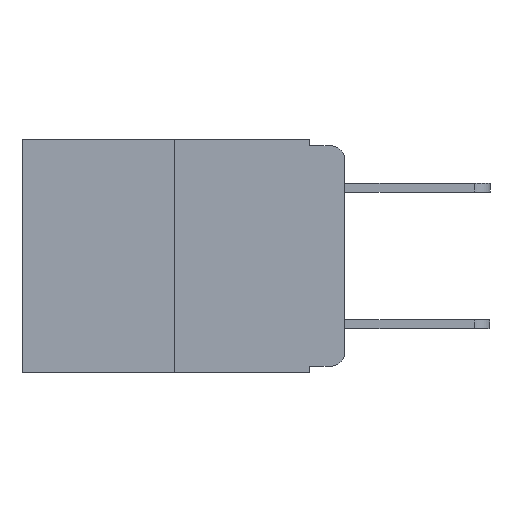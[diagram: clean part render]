
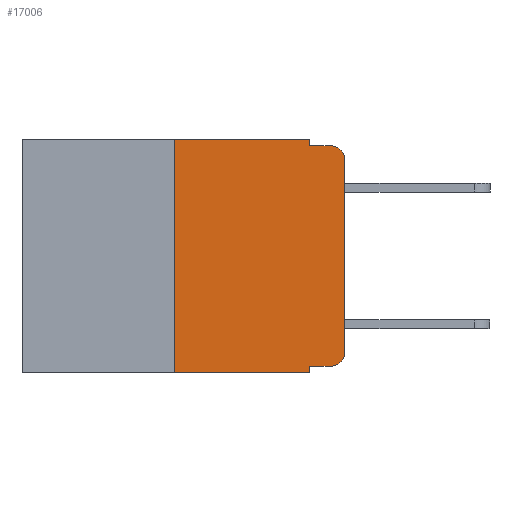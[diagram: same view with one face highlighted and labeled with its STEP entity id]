
A CAD part, left-side view. The second image highlights one B-rep face of the part: STEP entity #17006.
In plain terms, the highlighted planar face has unit normal (-1, 0, 0).
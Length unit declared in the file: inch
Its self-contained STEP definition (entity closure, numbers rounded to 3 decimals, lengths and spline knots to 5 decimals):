
#28 = DIRECTION ( 'NONE',  ( 0., 0., 1. ) ) ;
#398 = EDGE_CURVE ( 'NONE', #14996, #5496, #13515, .T. ) ;
#632 = CARTESIAN_POINT ( 'NONE',  ( 0., 0., 0. ) ) ;
#847 = EDGE_CURVE ( 'NONE', #13407, #10683, #22896, .T. ) ;
#879 = CARTESIAN_POINT ( 'NONE',  ( 0., 0.051, 0. ) ) ;
#947 = ORIENTED_EDGE ( 'NONE', *, *, #847, .F. ) ;
#1646 = VECTOR ( 'NONE', #8647, 39.37008 ) ;
#2410 = CARTESIAN_POINT ( 'NONE',  ( 0., 0.02, -0.313 ) ) ;
#2514 = AXIS2_PLACEMENT_3D ( 'NONE', #2410, #15236, #4352 ) ;
#2531 = CARTESIAN_POINT ( 'NONE',  ( 0., 0.473, -0.343 ) ) ;
#2875 = CARTESIAN_POINT ( 'NONE',  ( 0., 0.25, 0. ) ) ;
#2968 = VERTEX_POINT ( 'NONE', #19376 ) ;
#3400 = PLANE ( 'NONE',  #21052 ) ;
#3443 = EDGE_CURVE ( 'NONE', #10683, #14114, #18419, .T. ) ;
#3958 = VECTOR ( 'NONE', #11970, 39.37008 ) ;
#4352 = DIRECTION ( 'NONE',  ( 0., 0., -1. ) ) ;
#4741 = EDGE_CURVE ( 'NONE', #15230, #14114, #15304, .T. ) ;
#5105 = VECTOR ( 'NONE', #18963, 39.37008 ) ;
#5323 = DIRECTION ( 'NONE',  ( 0., 0., -1. ) ) ;
#5496 = VERTEX_POINT ( 'NONE', #22083 ) ;
#5988 = EDGE_CURVE ( 'NONE', #2968, #15230, #6943, .T. ) ;
#6168 = CARTESIAN_POINT ( 'NONE',  ( 0., 0.051, -0.333 ) ) ;
#6943 = LINE ( 'NONE', #632, #15933 ) ;
#8115 = CARTESIAN_POINT ( 'NONE',  ( 0., 0.051, -0.01 ) ) ;
#8647 = DIRECTION ( 'NONE',  ( 0., 0., 1. ) ) ;
#9089 = EDGE_CURVE ( 'NONE', #20933, #13407, #13251, .T. ) ;
#10307 = ORIENTED_EDGE ( 'NONE', *, *, #4741, .T. ) ;
#10341 = VECTOR ( 'NONE', #21793, 39.37008 ) ;
#10683 = VERTEX_POINT ( 'NONE', #8115 ) ;
#10888 = LINE ( 'NONE', #14692, #10341 ) ;
#11970 = DIRECTION ( 'NONE',  ( 0., -1., 0. ) ) ;
#12335 = CARTESIAN_POINT ( 'NONE',  ( 0., 0.473, 0. ) ) ;
#12563 = ORIENTED_EDGE ( 'NONE', *, *, #23173, .F. ) ;
#12940 = VECTOR ( 'NONE', #14552, 39.37008 ) ;
#13251 = LINE ( 'NONE', #12335, #22099 ) ;
#13407 = VERTEX_POINT ( 'NONE', #23140 ) ;
#13515 = LINE ( 'NONE', #2531, #12940 ) ;
#13629 = CIRCLE ( 'NONE', #2514, 0.02 ) ;
#14063 = VECTOR ( 'NONE', #23509, 39.37008 ) ;
#14114 = VERTEX_POINT ( 'NONE', #19898 ) ;
#14155 = DIRECTION ( 'NONE',  ( 0., -1., 0. ) ) ;
#14428 = CARTESIAN_POINT ( 'NONE',  ( 0., 0., -0.03 ) ) ;
#14552 = DIRECTION ( 'NONE',  ( 0., -1., 0. ) ) ;
#14692 = CARTESIAN_POINT ( 'NONE',  ( 0., 0.051, -0.333 ) ) ;
#14815 = ORIENTED_EDGE ( 'NONE', *, *, #16123, .T. ) ;
#14996 = VERTEX_POINT ( 'NONE', #22612 ) ;
#15088 = ORIENTED_EDGE ( 'NONE', *, *, #3443, .F. ) ;
#15230 = VERTEX_POINT ( 'NONE', #14428 ) ;
#15236 = DIRECTION ( 'NONE',  ( -1., 0., 0. ) ) ;
#15304 = CIRCLE ( 'NONE', #21744, 0.02 ) ;
#15377 = CARTESIAN_POINT ( 'NONE',  ( 0., 0.051, 0. ) ) ;
#15645 = CARTESIAN_POINT ( 'NONE',  ( 0., 0.02, -0.333 ) ) ;
#15814 = CARTESIAN_POINT ( 'NONE',  ( 0., 0.25, 0. ) ) ;
#15933 = VECTOR ( 'NONE', #28, 39.37008 ) ;
#16123 = EDGE_CURVE ( 'NONE', #16305, #2968, #13629, .T. ) ;
#16161 = DIRECTION ( 'NONE',  ( 1., 0., 0. ) ) ;
#16305 = VERTEX_POINT ( 'NONE', #15645 ) ;
#17006 = ADVANCED_FACE ( 'NONE', ( #21324 ), #3400, .F. ) ;
#17874 = CARTESIAN_POINT ( 'NONE',  ( 0., 0.473, 0. ) ) ;
#18419 = LINE ( 'NONE', #22889, #3958 ) ;
#18437 = ORIENTED_EDGE ( 'NONE', *, *, #20854, .F. ) ;
#18493 = EDGE_CURVE ( 'NONE', #18655, #16305, #10888, .T. ) ;
#18655 = VERTEX_POINT ( 'NONE', #6168 ) ;
#18723 = ORIENTED_EDGE ( 'NONE', *, *, #5988, .T. ) ;
#18963 = DIRECTION ( 'NONE',  ( 0., 0., -1. ) ) ;
#19376 = CARTESIAN_POINT ( 'NONE',  ( 0., 0., -0.313 ) ) ;
#19471 = LINE ( 'NONE', #15377, #5105 ) ;
#19898 = CARTESIAN_POINT ( 'NONE',  ( 0., 0.02, -0.01 ) ) ;
#20854 = EDGE_CURVE ( 'NONE', #18655, #5496, #19471, .T. ) ;
#20909 = ORIENTED_EDGE ( 'NONE', *, *, #9089, .F. ) ;
#20933 = VERTEX_POINT ( 'NONE', #2875 ) ;
#21011 = LINE ( 'NONE', #15814, #1646 ) ;
#21052 = AXIS2_PLACEMENT_3D ( 'NONE', #17874, #16161, #5323 ) ;
#21324 = FACE_OUTER_BOUND ( 'NONE', #22911, .T. ) ;
#21744 = AXIS2_PLACEMENT_3D ( 'NONE', #23252, #23149, #23101 ) ;
#21793 = DIRECTION ( 'NONE',  ( 0., -1., 0. ) ) ;
#21981 = ORIENTED_EDGE ( 'NONE', *, *, #398, .T. ) ;
#22083 = CARTESIAN_POINT ( 'NONE',  ( 0., 0.051, -0.343 ) ) ;
#22099 = VECTOR ( 'NONE', #14155, 39.37008 ) ;
#22612 = CARTESIAN_POINT ( 'NONE',  ( 0., 0.25, -0.343 ) ) ;
#22889 = CARTESIAN_POINT ( 'NONE',  ( 0., 0.051, -0.01 ) ) ;
#22896 = LINE ( 'NONE', #879, #14063 ) ;
#22911 = EDGE_LOOP ( 'NONE', ( #18723, #10307, #15088, #947, #20909, #12563, #21981, #18437, #23091, #14815 ) ) ;
#23091 = ORIENTED_EDGE ( 'NONE', *, *, #18493, .T. ) ;
#23101 = DIRECTION ( 'NONE',  ( 0., 0., -1. ) ) ;
#23140 = CARTESIAN_POINT ( 'NONE',  ( 0., 0.051, 0. ) ) ;
#23149 = DIRECTION ( 'NONE',  ( -1., 0., 0. ) ) ;
#23173 = EDGE_CURVE ( 'NONE', #14996, #20933, #21011, .T. ) ;
#23252 = CARTESIAN_POINT ( 'NONE',  ( 0., 0.02, -0.03 ) ) ;
#23509 = DIRECTION ( 'NONE',  ( 0., 0., -1. ) ) ;
